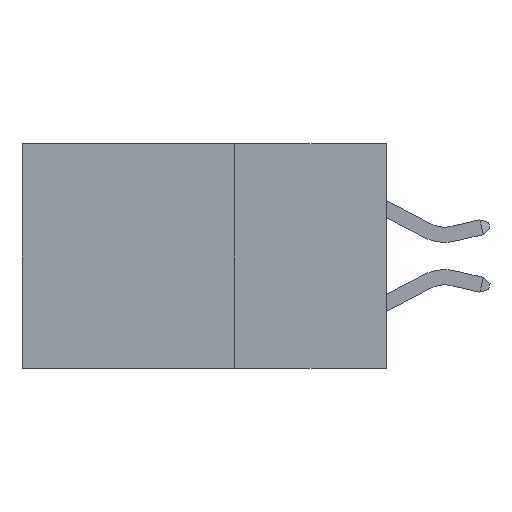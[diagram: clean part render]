
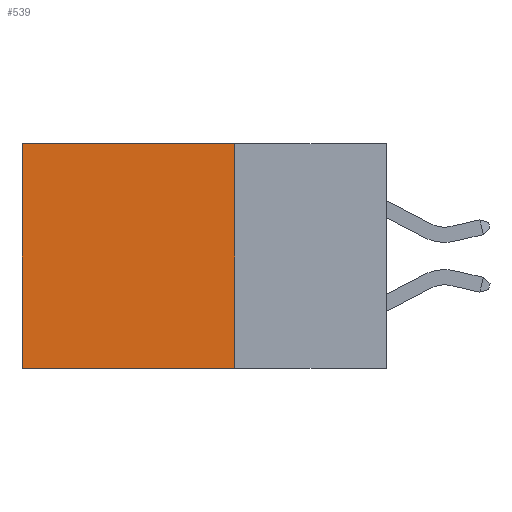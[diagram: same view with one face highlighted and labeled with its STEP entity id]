
A CAD part, left-side view. The second image highlights one B-rep face of the part: STEP entity #539.
In plain terms, the highlighted planar face has unit normal (-1, 0, 0).
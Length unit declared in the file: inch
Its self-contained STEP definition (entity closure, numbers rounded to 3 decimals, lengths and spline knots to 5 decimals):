
#362 = DIRECTION ( 'NONE',  ( 0., 0., -1. ) ) ;
#407 = CARTESIAN_POINT ( 'NONE',  ( 0.2615, 0.6, -0.37 ) ) ;
#539 = ADVANCED_FACE ( 'NONE', ( #3807 ), #5944, .F. ) ;
#819 = EDGE_CURVE ( 'NONE', #4636, #10614, #10328, .T. ) ;
#1190 = LINE ( 'NONE', #4480, #5803 ) ;
#1351 = VECTOR ( 'NONE', #362, 39.37008 ) ;
#1446 = VECTOR ( 'NONE', #2951, 39.37008 ) ;
#1717 = EDGE_CURVE ( 'NONE', #10302, #7353, #6018, .T. ) ;
#1866 = ORIENTED_EDGE ( 'NONE', *, *, #6194, .T. ) ;
#2300 = EDGE_LOOP ( 'NONE', ( #1866, #6380, #8521, #6654 ) ) ;
#2737 = DIRECTION ( 'NONE',  ( 0., 0., -1. ) ) ;
#2951 = DIRECTION ( 'NONE',  ( 0., 1., 0. ) ) ;
#3807 = FACE_OUTER_BOUND ( 'NONE', #2300, .T. ) ;
#4313 = CARTESIAN_POINT ( 'NONE',  ( 0.2615, 0.25, 0. ) ) ;
#4462 = CARTESIAN_POINT ( 'NONE',  ( 0.2615, 0.25, -0.37 ) ) ;
#4480 = CARTESIAN_POINT ( 'NONE',  ( 0.2615, 0.25, -0.37 ) ) ;
#4636 = VERTEX_POINT ( 'NONE', #4313 ) ;
#5469 = AXIS2_PLACEMENT_3D ( 'NONE', #5995, #9807, #2737 ) ;
#5803 = VECTOR ( 'NONE', #7754, 39.37008 ) ;
#5944 = PLANE ( 'NONE',  #5469 ) ;
#5995 = CARTESIAN_POINT ( 'NONE',  ( 0.2615, 0.25, -0.37 ) ) ;
#6018 = LINE ( 'NONE', #4462, #1446 ) ;
#6194 = EDGE_CURVE ( 'NONE', #10614, #7353, #8108, .T. ) ;
#6284 = CARTESIAN_POINT ( 'NONE',  ( 0.2615, 0.6, -0.37 ) ) ;
#6380 = ORIENTED_EDGE ( 'NONE', *, *, #1717, .F. ) ;
#6654 = ORIENTED_EDGE ( 'NONE', *, *, #819, .T. ) ;
#7095 = CARTESIAN_POINT ( 'NONE',  ( 0.2615, 0.25, -0.37 ) ) ;
#7353 = VERTEX_POINT ( 'NONE', #6284 ) ;
#7754 = DIRECTION ( 'NONE',  ( 0., 0., -1. ) ) ;
#7942 = EDGE_CURVE ( 'NONE', #4636, #10302, #1190, .T. ) ;
#8108 = LINE ( 'NONE', #407, #1351 ) ;
#8295 = VECTOR ( 'NONE', #9384, 39.37008 ) ;
#8521 = ORIENTED_EDGE ( 'NONE', *, *, #7942, .F. ) ;
#9134 = CARTESIAN_POINT ( 'NONE',  ( 0.2615, 0.25, 0. ) ) ;
#9384 = DIRECTION ( 'NONE',  ( 0., 1., 0. ) ) ;
#9626 = CARTESIAN_POINT ( 'NONE',  ( 0.2615, 0.6, 0. ) ) ;
#9807 = DIRECTION ( 'NONE',  ( 1., 0., 0. ) ) ;
#10302 = VERTEX_POINT ( 'NONE', #7095 ) ;
#10328 = LINE ( 'NONE', #9134, #8295 ) ;
#10614 = VERTEX_POINT ( 'NONE', #9626 ) ;
